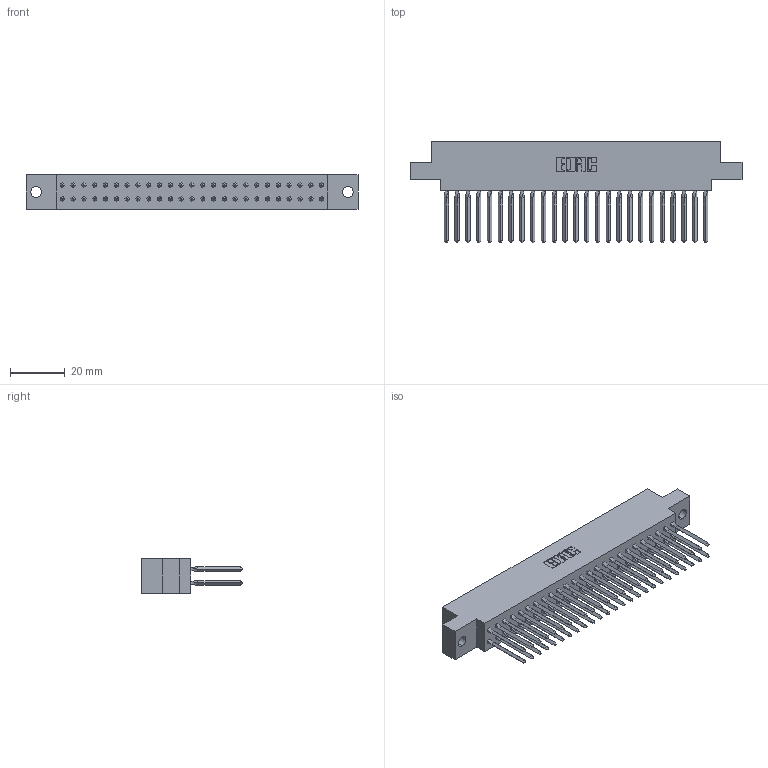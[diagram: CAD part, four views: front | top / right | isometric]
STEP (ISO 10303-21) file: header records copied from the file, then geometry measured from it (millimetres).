
FILE_DESCRIPTION (( 'STEP AP203' ), '1' );
FILE_NAME ('317-050-542-804.STEP', '2020-02-28T03:12:10', ( '' ), ( '' ), 'SwSTEP 2.0', 'SolidWorks 2016', '' );
FILE_SCHEMA (( 'CONFIG_CONTROL_DESIGN' ));
Length unit declared in the file: inch
Products named in the file (3): 317-050-542-804; 317 Part_.156 Dia - TH; 317-290-003_542
Assembly tree (51 placements, depth 2):
  317-050-542-804
    317 Part_.156 Dia - TH
    317-290-003_542  x50
Bounding box: 121.77 x 37.34 x 12.7 mm (x, y, z)
Volume: 19313.9 mm3; surface area: 26129.5 mm2
Topology: 51 solids, 51 shells, 2952 faces, 8275 edges, 5282 vertices
Faces by surface type: plane 2358, cylinder 394, bspline 200
Entity records: 37529 total; most frequent: CARTESIAN_POINT 6793, ORIENTED_EDGE 6456, DIRECTION 5460, EDGE_CURVE 3228, LINE 3058, VECTOR 3058, VERTEX_POINT 2146, AXIS2_PLACEMENT_3D 1201
